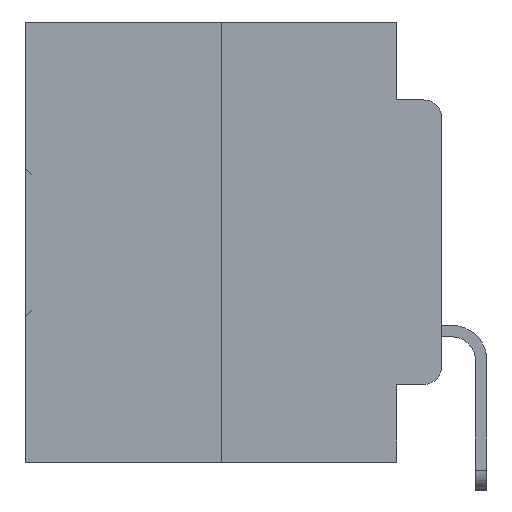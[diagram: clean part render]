
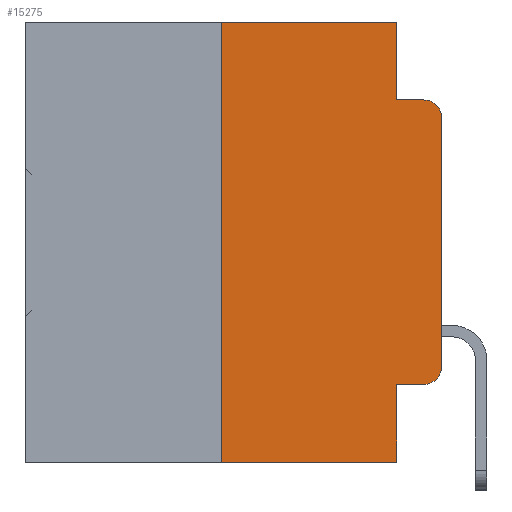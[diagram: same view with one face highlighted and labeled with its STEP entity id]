
A CAD part, left-side view. The second image highlights one B-rep face of the part: STEP entity #15275.
In plain terms, the highlighted planar face has unit normal (-1, 0, 0).
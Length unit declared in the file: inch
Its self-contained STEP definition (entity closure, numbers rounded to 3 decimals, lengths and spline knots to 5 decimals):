
#1314 = VECTOR ( 'NONE', #12027, 39.37008 ) ;
#1859 = CARTESIAN_POINT ( 'NONE',  ( 0., 0.051, -0.5 ) ) ;
#2090 = VECTOR ( 'NONE', #22637, 39.37008 ) ;
#2982 = LINE ( 'NONE', #15202, #23712 ) ;
#3954 = ORIENTED_EDGE ( 'NONE', *, *, #16588, .F. ) ;
#4385 = CARTESIAN_POINT ( 'NONE',  ( 0., 0.25, 0. ) ) ;
#4675 = DIRECTION ( 'NONE',  ( 0., 0., -1. ) ) ;
#4889 = ORIENTED_EDGE ( 'NONE', *, *, #17161, .F. ) ;
#5429 = CARTESIAN_POINT ( 'NONE',  ( 0., 0.25, 0. ) ) ;
#6192 = EDGE_CURVE ( 'NONE', #8075, #26533, #26055, .T. ) ;
#6407 = VERTEX_POINT ( 'NONE', #33426 ) ;
#6649 = CARTESIAN_POINT ( 'NONE',  ( 0., 0.051, 0. ) ) ;
#7007 = CARTESIAN_POINT ( 'NONE',  ( 0., 0.02, -0.1085 ) ) ;
#8075 = VERTEX_POINT ( 'NONE', #19767 ) ;
#8168 = LINE ( 'NONE', #13092, #34010 ) ;
#8189 = DIRECTION ( 'NONE',  ( 0., 0., 1. ) ) ;
#9448 = DIRECTION ( 'NONE',  ( 0., -1., 0. ) ) ;
#9771 = DIRECTION ( 'NONE',  ( 0., 0., -1. ) ) ;
#9900 = EDGE_CURVE ( 'NONE', #13073, #8075, #12784, .T. ) ;
#10389 = FACE_OUTER_BOUND ( 'NONE', #29443, .T. ) ;
#10390 = DIRECTION ( 'NONE',  ( 0., -1., 0. ) ) ;
#10391 = VERTEX_POINT ( 'NONE', #17891 ) ;
#10510 = VECTOR ( 'NONE', #8189, 39.37008 ) ;
#10831 = ORIENTED_EDGE ( 'NONE', *, *, #15112, .T. ) ;
#11591 = CARTESIAN_POINT ( 'NONE',  ( 0., 0.051, -0.0885 ) ) ;
#11607 = DIRECTION ( 'NONE',  ( -1., 0., 0. ) ) ;
#12027 = DIRECTION ( 'NONE',  ( 0., 0., -1. ) ) ;
#12784 = LINE ( 'NONE', #32548, #31494 ) ;
#12946 = ORIENTED_EDGE ( 'NONE', *, *, #20741, .F. ) ;
#13073 = VERTEX_POINT ( 'NONE', #27210 ) ;
#13092 = CARTESIAN_POINT ( 'NONE',  ( 0., 0.473, 0. ) ) ;
#15112 = EDGE_CURVE ( 'NONE', #6407, #34649, #20970, .T. ) ;
#15202 = CARTESIAN_POINT ( 'NONE',  ( 0., 0.051, 0. ) ) ;
#15275 = ADVANCED_FACE ( 'NONE', ( #10389 ), #33988, .F. ) ;
#15931 = LINE ( 'NONE', #6649, #1314 ) ;
#16274 = ORIENTED_EDGE ( 'NONE', *, *, #31311, .T. ) ;
#16451 = CARTESIAN_POINT ( 'NONE',  ( 0., 0., 0. ) ) ;
#16588 = EDGE_CURVE ( 'NONE', #23265, #32692, #8168, .T. ) ;
#16857 = VECTOR ( 'NONE', #21737, 39.37008 ) ;
#17161 = EDGE_CURVE ( 'NONE', #13073, #34649, #2982, .T. ) ;
#17230 = ORIENTED_EDGE ( 'NONE', *, *, #9900, .T. ) ;
#17891 = CARTESIAN_POINT ( 'NONE',  ( 0., 0.02, -0.0885 ) ) ;
#17960 = CARTESIAN_POINT ( 'NONE',  ( 0., 0., -0.1085 ) ) ;
#17975 = DIRECTION ( 'NONE',  ( 0., 0., -1. ) ) ;
#18215 = CARTESIAN_POINT ( 'NONE',  ( 0., 0.473, 0. ) ) ;
#19455 = DIRECTION ( 'NONE',  ( 0., -1., 0. ) ) ;
#19767 = CARTESIAN_POINT ( 'NONE',  ( 0., 0.02, -0.4115 ) ) ;
#20001 = CARTESIAN_POINT ( 'NONE',  ( 0., 0.051, -0.0885 ) ) ;
#20498 = AXIS2_PLACEMENT_3D ( 'NONE', #18215, #20909, #4675 ) ;
#20741 = EDGE_CURVE ( 'NONE', #6407, #23265, #31762, .T. ) ;
#20909 = DIRECTION ( 'NONE',  ( 1., 0., 0. ) ) ;
#20970 = LINE ( 'NONE', #28129, #28779 ) ;
#21737 = DIRECTION ( 'NONE',  ( 0., 0., 1. ) ) ;
#22516 = EDGE_CURVE ( 'NONE', #32692, #30595, #15931, .T. ) ;
#22637 = DIRECTION ( 'NONE',  ( 0., -1., 0. ) ) ;
#22963 = ORIENTED_EDGE ( 'NONE', *, *, #22516, .F. ) ;
#23265 = VERTEX_POINT ( 'NONE', #4385 ) ;
#23712 = VECTOR ( 'NONE', #17975, 39.37008 ) ;
#24272 = EDGE_CURVE ( 'NONE', #30595, #10391, #24535, .T. ) ;
#24535 = LINE ( 'NONE', #20001, #2090 ) ;
#24989 = ORIENTED_EDGE ( 'NONE', *, *, #24272, .F. ) ;
#25806 = DIRECTION ( 'NONE',  ( -1., 0., 0. ) ) ;
#25990 = AXIS2_PLACEMENT_3D ( 'NONE', #27588, #11607, #30238 ) ;
#26055 = CIRCLE ( 'NONE', #25990, 0.02 ) ;
#26533 = VERTEX_POINT ( 'NONE', #31680 ) ;
#26902 = CIRCLE ( 'NONE', #32044, 0.02 ) ;
#27210 = CARTESIAN_POINT ( 'NONE',  ( 0., 0.051, -0.4115 ) ) ;
#27588 = CARTESIAN_POINT ( 'NONE',  ( 0., 0.02, -0.3915 ) ) ;
#28129 = CARTESIAN_POINT ( 'NONE',  ( 0., 0.473, -0.5 ) ) ;
#28164 = CARTESIAN_POINT ( 'NONE',  ( 0., 0.051, 0. ) ) ;
#28259 = ORIENTED_EDGE ( 'NONE', *, *, #33059, .T. ) ;
#28779 = VECTOR ( 'NONE', #9448, 39.37008 ) ;
#28899 = VERTEX_POINT ( 'NONE', #17960 ) ;
#29443 = EDGE_LOOP ( 'NONE', ( #28259, #16274, #24989, #22963, #3954, #12946, #10831, #4889, #17230, #32921 ) ) ;
#30238 = DIRECTION ( 'NONE',  ( 0., 0., -1. ) ) ;
#30595 = VERTEX_POINT ( 'NONE', #11591 ) ;
#30918 = LINE ( 'NONE', #16451, #16857 ) ;
#31311 = EDGE_CURVE ( 'NONE', #28899, #10391, #26902, .T. ) ;
#31494 = VECTOR ( 'NONE', #19455, 39.37008 ) ;
#31680 = CARTESIAN_POINT ( 'NONE',  ( 0., 0., -0.3915 ) ) ;
#31762 = LINE ( 'NONE', #5429, #10510 ) ;
#32044 = AXIS2_PLACEMENT_3D ( 'NONE', #7007, #25806, #9771 ) ;
#32548 = CARTESIAN_POINT ( 'NONE',  ( 0., 0.051, -0.4115 ) ) ;
#32692 = VERTEX_POINT ( 'NONE', #28164 ) ;
#32921 = ORIENTED_EDGE ( 'NONE', *, *, #6192, .T. ) ;
#33059 = EDGE_CURVE ( 'NONE', #26533, #28899, #30918, .T. ) ;
#33426 = CARTESIAN_POINT ( 'NONE',  ( 0., 0.25, -0.5 ) ) ;
#33988 = PLANE ( 'NONE',  #20498 ) ;
#34010 = VECTOR ( 'NONE', #10390, 39.37008 ) ;
#34649 = VERTEX_POINT ( 'NONE', #1859 ) ;
